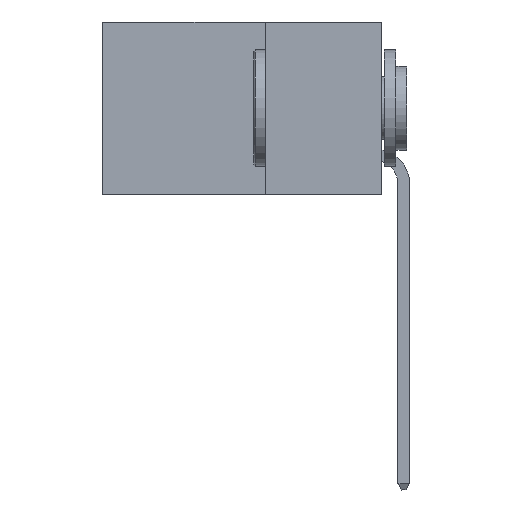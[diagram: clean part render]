
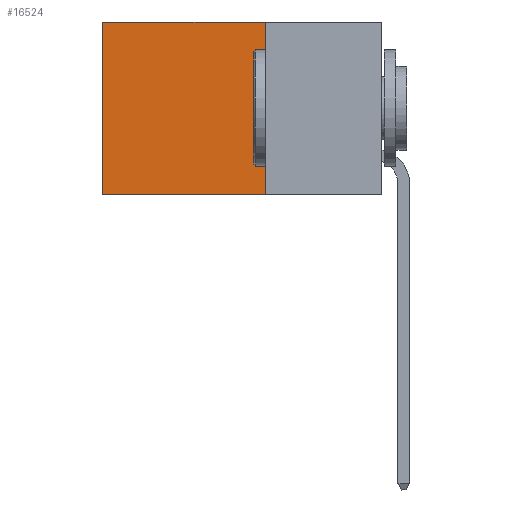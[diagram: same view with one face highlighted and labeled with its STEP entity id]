
A CAD part, left-side view. The second image highlights one B-rep face of the part: STEP entity #16524.
In plain terms, the highlighted planar face has unit normal (-1, 0, 0).
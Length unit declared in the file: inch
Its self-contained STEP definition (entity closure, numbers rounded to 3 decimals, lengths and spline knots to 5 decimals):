
#212 = VERTEX_POINT ( 'NONE', #20993 ) ;
#821 = PLANE ( 'NONE',  #3715 ) ;
#918 = LINE ( 'NONE', #18718, #13427 ) ;
#3715 = AXIS2_PLACEMENT_3D ( 'NONE', #5864, #23307, #8343 ) ;
#5864 = CARTESIAN_POINT ( 'NONE',  ( 0.2875, 0.25, 0. ) ) ;
#6350 = CARTESIAN_POINT ( 'NONE',  ( 0.2875, 0.25, -0.37 ) ) ;
#8057 = LINE ( 'NONE', #29449, #8839 ) ;
#8343 = DIRECTION ( 'NONE',  ( 0., 0., -1. ) ) ;
#8554 = VECTOR ( 'NONE', #31195, 39.37008 ) ;
#8800 = EDGE_CURVE ( 'NONE', #14092, #8902, #10440, .T. ) ;
#8839 = VECTOR ( 'NONE', #17051, 39.37008 ) ;
#8902 = VERTEX_POINT ( 'NONE', #6350 ) ;
#10440 = LINE ( 'NONE', #20992, #17180 ) ;
#13427 = VECTOR ( 'NONE', #21333, 39.37008 ) ;
#13562 = CARTESIAN_POINT ( 'NONE',  ( 0.2875, 0.6, -0.37 ) ) ;
#14092 = VERTEX_POINT ( 'NONE', #26379 ) ;
#14731 = EDGE_CURVE ( 'NONE', #212, #17945, #918, .T. ) ;
#15707 = ORIENTED_EDGE ( 'NONE', *, *, #22638, .F. ) ;
#16524 = ADVANCED_FACE ( 'NONE', ( #19613 ), #821, .F. ) ;
#17051 = DIRECTION ( 'NONE',  ( 0., 1., 0. ) ) ;
#17180 = VECTOR ( 'NONE', #23479, 39.37008 ) ;
#17945 = VERTEX_POINT ( 'NONE', #13562 ) ;
#18718 = CARTESIAN_POINT ( 'NONE',  ( 0.2875, 0.6, 0. ) ) ;
#19396 = ORIENTED_EDGE ( 'NONE', *, *, #14731, .T. ) ;
#19613 = FACE_OUTER_BOUND ( 'NONE', #28087, .T. ) ;
#20475 = EDGE_CURVE ( 'NONE', #14092, #212, #21868, .T. ) ;
#20992 = CARTESIAN_POINT ( 'NONE',  ( 0.2875, 0.25, 0. ) ) ;
#20993 = CARTESIAN_POINT ( 'NONE',  ( 0.2875, 0.6, 0. ) ) ;
#21333 = DIRECTION ( 'NONE',  ( 0., 0., -1. ) ) ;
#21705 = ORIENTED_EDGE ( 'NONE', *, *, #20475, .T. ) ;
#21868 = LINE ( 'NONE', #28699, #8554 ) ;
#22638 = EDGE_CURVE ( 'NONE', #8902, #17945, #8057, .T. ) ;
#23307 = DIRECTION ( 'NONE',  ( 1., 0., 0. ) ) ;
#23479 = DIRECTION ( 'NONE',  ( 0., 0., -1. ) ) ;
#26379 = CARTESIAN_POINT ( 'NONE',  ( 0.2875, 0.25, 0. ) ) ;
#28087 = EDGE_LOOP ( 'NONE', ( #19396, #15707, #31802, #21705 ) ) ;
#28699 = CARTESIAN_POINT ( 'NONE',  ( 0.2875, 0.25, 0. ) ) ;
#29449 = CARTESIAN_POINT ( 'NONE',  ( 0.2875, 0.25, -0.37 ) ) ;
#31195 = DIRECTION ( 'NONE',  ( 0., 1., 0. ) ) ;
#31802 = ORIENTED_EDGE ( 'NONE', *, *, #8800, .F. ) ;
